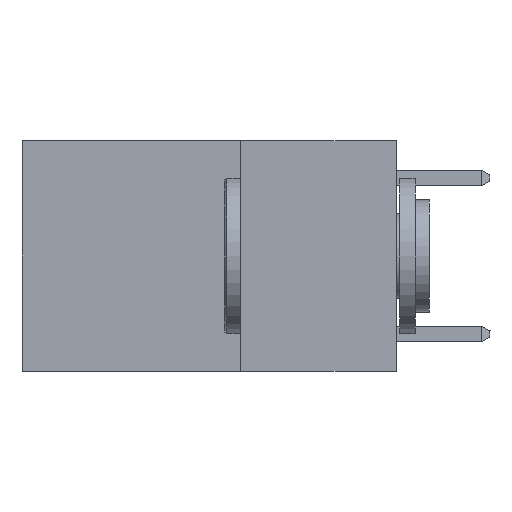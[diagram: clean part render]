
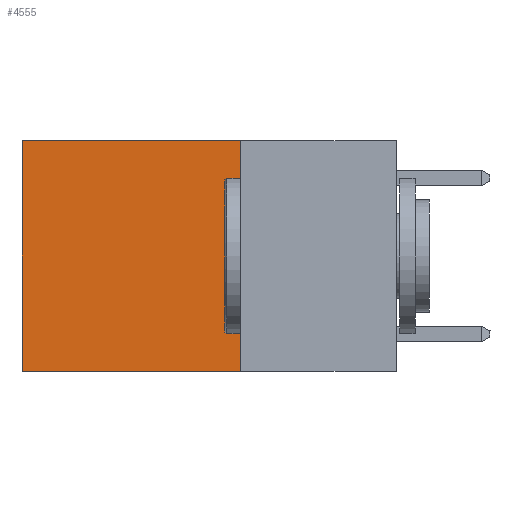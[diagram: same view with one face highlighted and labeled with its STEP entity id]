
A CAD part, left-side view. The second image highlights one B-rep face of the part: STEP entity #4555.
In plain terms, the highlighted planar face has unit normal (-1, 0, 0).
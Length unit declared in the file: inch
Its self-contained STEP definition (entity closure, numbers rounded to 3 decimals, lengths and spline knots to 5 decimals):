
#386 = VERTEX_POINT ( 'NONE', #8195 ) ;
#1448 = VECTOR ( 'NONE', #9247, 39.37008 ) ;
#1692 = LINE ( 'NONE', #14743, #2120 ) ;
#2085 = LINE ( 'NONE', #15889, #1448 ) ;
#2120 = VECTOR ( 'NONE', #16196, 39.37008 ) ;
#2206 = CARTESIAN_POINT ( 'NONE',  ( 0.2625, 0.25, -0.37 ) ) ;
#4555 = ADVANCED_FACE ( 'NONE', ( #13968 ), #9770, .F. ) ;
#4624 = CARTESIAN_POINT ( 'NONE',  ( 0.2625, 0.25, 0. ) ) ;
#4701 = CARTESIAN_POINT ( 'NONE',  ( 0.2625, 0.6, 0. ) ) ;
#5677 = VERTEX_POINT ( 'NONE', #5862 ) ;
#5862 = CARTESIAN_POINT ( 'NONE',  ( 0.2625, 0.6, 0. ) ) ;
#5911 = DIRECTION ( 'NONE',  ( 0., 0., -1. ) ) ;
#6174 = VECTOR ( 'NONE', #12357, 39.37008 ) ;
#6377 = EDGE_CURVE ( 'NONE', #5677, #13001, #15975, .T. ) ;
#7102 = CARTESIAN_POINT ( 'NONE',  ( 0.2625, 0.25, 0. ) ) ;
#7592 = ORIENTED_EDGE ( 'NONE', *, *, #15863, .F. ) ;
#8195 = CARTESIAN_POINT ( 'NONE',  ( 0.2625, 0.25, 0. ) ) ;
#8292 = ORIENTED_EDGE ( 'NONE', *, *, #6377, .T. ) ;
#9180 = ORIENTED_EDGE ( 'NONE', *, *, #12248, .F. ) ;
#9247 = DIRECTION ( 'NONE',  ( 0., 1., 0. ) ) ;
#9770 = PLANE ( 'NONE',  #12457 ) ;
#10130 = LINE ( 'NONE', #4624, #6174 ) ;
#10922 = EDGE_LOOP ( 'NONE', ( #8292, #9180, #7592, #17046 ) ) ;
#11562 = EDGE_CURVE ( 'NONE', #386, #5677, #1692, .T. ) ;
#12248 = EDGE_CURVE ( 'NONE', #14793, #13001, #2085, .T. ) ;
#12357 = DIRECTION ( 'NONE',  ( 0., 0., -1. ) ) ;
#12457 = AXIS2_PLACEMENT_3D ( 'NONE', #7102, #12470, #16477 ) ;
#12470 = DIRECTION ( 'NONE',  ( 1., 0., 0. ) ) ;
#13001 = VERTEX_POINT ( 'NONE', #14133 ) ;
#13463 = VECTOR ( 'NONE', #5911, 39.37008 ) ;
#13968 = FACE_OUTER_BOUND ( 'NONE', #10922, .T. ) ;
#14133 = CARTESIAN_POINT ( 'NONE',  ( 0.2625, 0.6, -0.37 ) ) ;
#14743 = CARTESIAN_POINT ( 'NONE',  ( 0.2625, 0.25, 0. ) ) ;
#14793 = VERTEX_POINT ( 'NONE', #2206 ) ;
#15863 = EDGE_CURVE ( 'NONE', #386, #14793, #10130, .T. ) ;
#15889 = CARTESIAN_POINT ( 'NONE',  ( 0.2625, 0.25, -0.37 ) ) ;
#15975 = LINE ( 'NONE', #4701, #13463 ) ;
#16196 = DIRECTION ( 'NONE',  ( 0., 1., 0. ) ) ;
#16477 = DIRECTION ( 'NONE',  ( 0., 0., -1. ) ) ;
#17046 = ORIENTED_EDGE ( 'NONE', *, *, #11562, .T. ) ;
